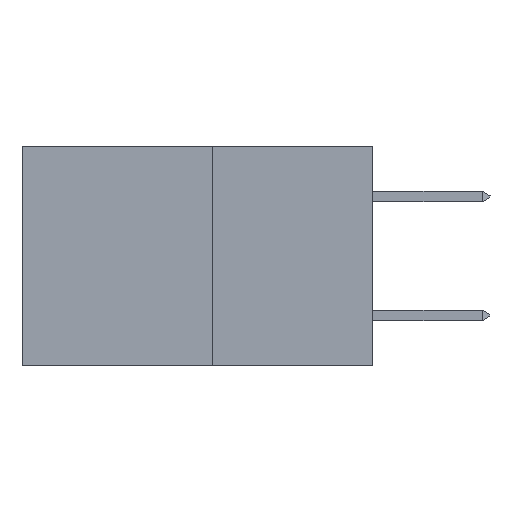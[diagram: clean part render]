
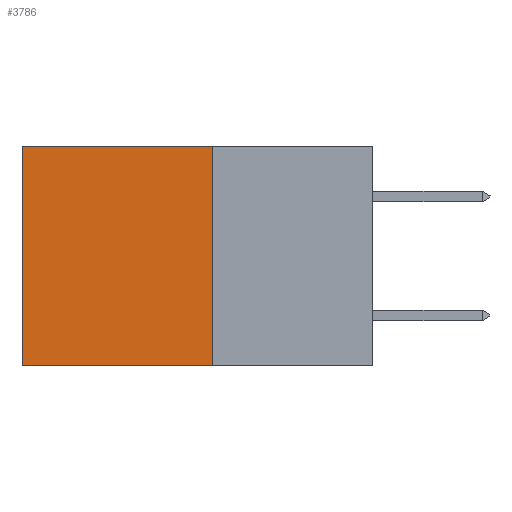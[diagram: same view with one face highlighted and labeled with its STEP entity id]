
A CAD part, left-side view. The second image highlights one B-rep face of the part: STEP entity #3786.
In plain terms, the highlighted planar face has unit normal (-1, 0, 0).
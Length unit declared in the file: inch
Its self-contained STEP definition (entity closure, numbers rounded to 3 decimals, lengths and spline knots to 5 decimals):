
#31 = CARTESIAN_POINT ( 'NONE',  ( 0.277, 0.59, 0. ) ) ;
#140 = EDGE_CURVE ( 'NONE', #6596, #9323, #9289, .T. ) ;
#343 = LINE ( 'NONE', #8743, #4434 ) ;
#473 = ORIENTED_EDGE ( 'NONE', *, *, #3401, .T. ) ;
#1076 = PLANE ( 'NONE',  #6501 ) ;
#1100 = LINE ( 'NONE', #5930, #7262 ) ;
#1110 = VECTOR ( 'NONE', #1753, 39.37008 ) ;
#1323 = FACE_OUTER_BOUND ( 'NONE', #8080, .T. ) ;
#1337 = CARTESIAN_POINT ( 'NONE',  ( 0.277, 0.59, -0.37 ) ) ;
#1414 = CARTESIAN_POINT ( 'NONE',  ( 0.277, 0.59, -0.37 ) ) ;
#1753 = DIRECTION ( 'NONE',  ( 0., 0., -1. ) ) ;
#2490 = EDGE_CURVE ( 'NONE', #6596, #4271, #1100, .T. ) ;
#2676 = ORIENTED_EDGE ( 'NONE', *, *, #7627, .F. ) ;
#2780 = DIRECTION ( 'NONE',  ( 1., 0., 0. ) ) ;
#3401 = EDGE_CURVE ( 'NONE', #4271, #8951, #9472, .T. ) ;
#3464 = DIRECTION ( 'NONE',  ( 0., 1., 0. ) ) ;
#3786 = ADVANCED_FACE ( 'NONE', ( #1323 ), #1076, .F. ) ;
#4271 = VERTEX_POINT ( 'NONE', #31 ) ;
#4434 = VECTOR ( 'NONE', #4888, 39.37008 ) ;
#4635 = CARTESIAN_POINT ( 'NONE',  ( 0.277, 0.27, 0. ) ) ;
#4888 = DIRECTION ( 'NONE',  ( 0., 1., 0. ) ) ;
#5143 = VECTOR ( 'NONE', #7759, 39.37008 ) ;
#5353 = CARTESIAN_POINT ( 'NONE',  ( 0.277, 0.27, -0.37 ) ) ;
#5930 = CARTESIAN_POINT ( 'NONE',  ( 0.277, 0.27, 0. ) ) ;
#6501 = AXIS2_PLACEMENT_3D ( 'NONE', #6710, #2780, #8277 ) ;
#6596 = VERTEX_POINT ( 'NONE', #4635 ) ;
#6710 = CARTESIAN_POINT ( 'NONE',  ( 0.277, 0.27, -0.37 ) ) ;
#6882 = ORIENTED_EDGE ( 'NONE', *, *, #140, .F. ) ;
#7262 = VECTOR ( 'NONE', #3464, 39.37008 ) ;
#7367 = CARTESIAN_POINT ( 'NONE',  ( 0.277, 0.27, -0.37 ) ) ;
#7627 = EDGE_CURVE ( 'NONE', #9323, #8951, #343, .T. ) ;
#7759 = DIRECTION ( 'NONE',  ( 0., 0., -1. ) ) ;
#8080 = EDGE_LOOP ( 'NONE', ( #473, #2676, #6882, #8910 ) ) ;
#8277 = DIRECTION ( 'NONE',  ( 0., 0., -1. ) ) ;
#8743 = CARTESIAN_POINT ( 'NONE',  ( 0.277, 0.27, -0.37 ) ) ;
#8910 = ORIENTED_EDGE ( 'NONE', *, *, #2490, .T. ) ;
#8951 = VERTEX_POINT ( 'NONE', #1414 ) ;
#9289 = LINE ( 'NONE', #5353, #1110 ) ;
#9323 = VERTEX_POINT ( 'NONE', #7367 ) ;
#9472 = LINE ( 'NONE', #1337, #5143 ) ;
